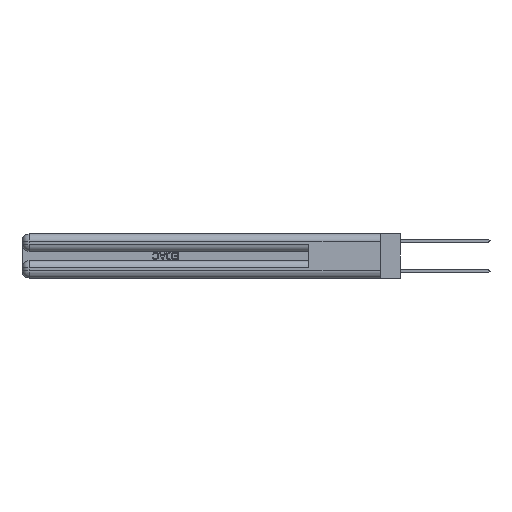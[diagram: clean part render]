
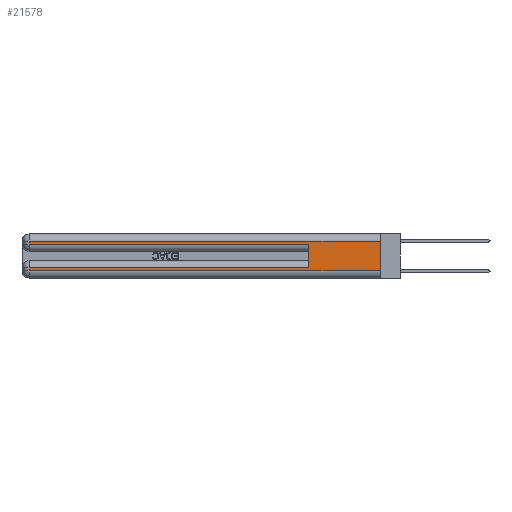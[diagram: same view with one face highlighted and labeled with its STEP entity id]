
A CAD part, left-side view. The second image highlights one B-rep face of the part: STEP entity #21578.
In plain terms, the highlighted planar face has unit normal (-1, 0, 0).
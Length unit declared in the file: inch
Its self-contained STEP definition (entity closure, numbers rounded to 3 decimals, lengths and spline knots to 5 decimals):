
#96 = CARTESIAN_POINT ( 'NONE',  ( 0., 0., 0.06 ) ) ;
#172 = VERTEX_POINT ( 'NONE', #24198 ) ;
#1190 = VECTOR ( 'NONE', #23264, 39.37008 ) ;
#1243 = CARTESIAN_POINT ( 'NONE',  ( 0., 2.94, 0.37 ) ) ;
#1780 = VECTOR ( 'NONE', #26356, 39.37008 ) ;
#2141 = VERTEX_POINT ( 'NONE', #5365 ) ;
#2235 = VERTEX_POINT ( 'NONE', #96 ) ;
#2659 = VECTOR ( 'NONE', #6511, 39.37008 ) ;
#2787 = ORIENTED_EDGE ( 'NONE', *, *, #7247, .T. ) ;
#3619 = CARTESIAN_POINT ( 'NONE',  ( 0., 0., 0.37 ) ) ;
#4075 = DIRECTION ( 'NONE',  ( 1., 0., 0. ) ) ;
#4880 = DIRECTION ( 'NONE',  ( 0., -1., 0. ) ) ;
#5365 = CARTESIAN_POINT ( 'NONE',  ( 0., 0.6, 0.285 ) ) ;
#5515 = LINE ( 'NONE', #10371, #34456 ) ;
#5597 = VECTOR ( 'NONE', #29384, 39.37008 ) ;
#6006 = VERTEX_POINT ( 'NONE', #15962 ) ;
#6220 = ORIENTED_EDGE ( 'NONE', *, *, #15875, .T. ) ;
#6455 = LINE ( 'NONE', #1243, #5597 ) ;
#6511 = DIRECTION ( 'NONE',  ( 0., 0., 1. ) ) ;
#7247 = EDGE_CURVE ( 'NONE', #6006, #2235, #13251, .T. ) ;
#7662 = DIRECTION ( 'NONE',  ( 0., -1., 0. ) ) ;
#9164 = CARTESIAN_POINT ( 'NONE',  ( 0., 2.94, 0.37 ) ) ;
#9298 = CARTESIAN_POINT ( 'NONE',  ( 0., 0.6, 0.145 ) ) ;
#10104 = VERTEX_POINT ( 'NONE', #33562 ) ;
#10146 = LINE ( 'NONE', #9298, #2659 ) ;
#10371 = CARTESIAN_POINT ( 'NONE',  ( 0., 0., 0.31 ) ) ;
#10386 = FACE_OUTER_BOUND ( 'NONE', #17159, .T. ) ;
#11229 = EDGE_CURVE ( 'NONE', #10104, #2141, #25326, .T. ) ;
#11254 = AXIS2_PLACEMENT_3D ( 'NONE', #20898, #4075, #23707 ) ;
#13251 = LINE ( 'NONE', #16011, #34785 ) ;
#13863 = LINE ( 'NONE', #9164, #20478 ) ;
#15059 = EDGE_CURVE ( 'NONE', #23917, #2141, #10146, .T. ) ;
#15100 = PLANE ( 'NONE',  #11254 ) ;
#15108 = EDGE_CURVE ( 'NONE', #23917, #172, #24214, .T. ) ;
#15875 = EDGE_CURVE ( 'NONE', #172, #6006, #6455, .T. ) ;
#15962 = CARTESIAN_POINT ( 'NONE',  ( 0., 2.94, 0.06 ) ) ;
#16011 = CARTESIAN_POINT ( 'NONE',  ( 0., 0., 0.06 ) ) ;
#16561 = VERTEX_POINT ( 'NONE', #18821 ) ;
#17159 = EDGE_LOOP ( 'NONE', ( #26034, #27287, #29112, #31540, #20102, #29495, #6220, #2787 ) ) ;
#18821 = CARTESIAN_POINT ( 'NONE',  ( 0., 2.94, 0.31 ) ) ;
#19809 = VERTEX_POINT ( 'NONE', #21489 ) ;
#20102 = ORIENTED_EDGE ( 'NONE', *, *, #15059, .F. ) ;
#20478 = VECTOR ( 'NONE', #31620, 39.37008 ) ;
#20726 = EDGE_CURVE ( 'NONE', #19809, #2235, #23631, .T. ) ;
#20898 = CARTESIAN_POINT ( 'NONE',  ( 0., 0., 0.37 ) ) ;
#21489 = CARTESIAN_POINT ( 'NONE',  ( 0., 0., 0.31 ) ) ;
#21578 = ADVANCED_FACE ( 'NONE', ( #10386 ), #15100, .F. ) ;
#21702 = DIRECTION ( 'NONE',  ( 0., 1., 0. ) ) ;
#23192 = EDGE_CURVE ( 'NONE', #16561, #10104, #13863, .T. ) ;
#23264 = DIRECTION ( 'NONE',  ( 0., 0., -1. ) ) ;
#23631 = LINE ( 'NONE', #3619, #1190 ) ;
#23707 = DIRECTION ( 'NONE',  ( 0., 0., -1. ) ) ;
#23917 = VERTEX_POINT ( 'NONE', #34532 ) ;
#24198 = CARTESIAN_POINT ( 'NONE',  ( 0., 2.94, 0.085 ) ) ;
#24214 = LINE ( 'NONE', #34845, #1780 ) ;
#25326 = LINE ( 'NONE', #27262, #31938 ) ;
#26034 = ORIENTED_EDGE ( 'NONE', *, *, #20726, .F. ) ;
#26356 = DIRECTION ( 'NONE',  ( 0., 1., 0. ) ) ;
#27262 = CARTESIAN_POINT ( 'NONE',  ( 0., 0., 0.285 ) ) ;
#27287 = ORIENTED_EDGE ( 'NONE', *, *, #30180, .T. ) ;
#29112 = ORIENTED_EDGE ( 'NONE', *, *, #23192, .T. ) ;
#29384 = DIRECTION ( 'NONE',  ( 0., 0., -1. ) ) ;
#29495 = ORIENTED_EDGE ( 'NONE', *, *, #15108, .T. ) ;
#30180 = EDGE_CURVE ( 'NONE', #19809, #16561, #5515, .T. ) ;
#31540 = ORIENTED_EDGE ( 'NONE', *, *, #11229, .T. ) ;
#31620 = DIRECTION ( 'NONE',  ( 0., 0., -1. ) ) ;
#31938 = VECTOR ( 'NONE', #7662, 39.37008 ) ;
#33562 = CARTESIAN_POINT ( 'NONE',  ( 0., 2.94, 0.285 ) ) ;
#34456 = VECTOR ( 'NONE', #21702, 39.37008 ) ;
#34532 = CARTESIAN_POINT ( 'NONE',  ( 0., 0.6, 0.085 ) ) ;
#34785 = VECTOR ( 'NONE', #4880, 39.37008 ) ;
#34845 = CARTESIAN_POINT ( 'NONE',  ( 0., 0., 0.085 ) ) ;
